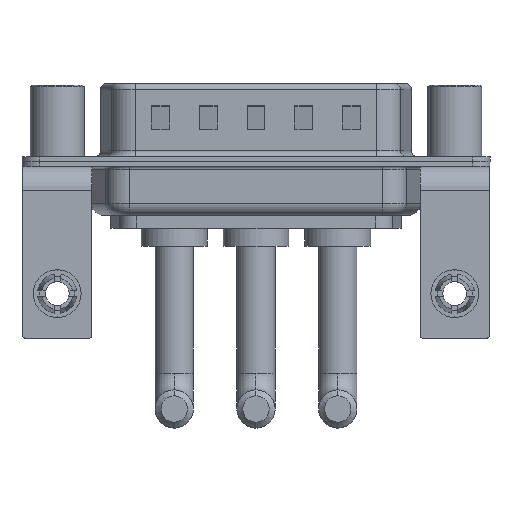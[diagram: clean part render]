
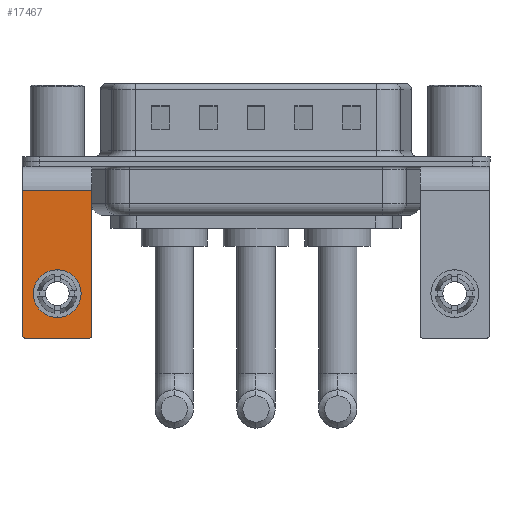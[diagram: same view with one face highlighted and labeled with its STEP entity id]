
A CAD part, front view. The second image highlights one B-rep face of the part: STEP entity #17467.
In plain terms, the highlighted planar face has unit normal (0, -1, 0).
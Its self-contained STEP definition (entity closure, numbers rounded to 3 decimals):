
#400 = DIRECTION ( 'NONE',  ( 0., 0., 1. ) ) ;
#445 = DIRECTION ( 'NONE',  ( -1., 0., 0. ) ) ;
#562 = CARTESIAN_POINT ( 'NONE',  ( -2.9, -6.25, -2.4 ) ) ;
#590 = VECTOR ( 'NONE', #445, 1000. ) ;
#670 = VERTEX_POINT ( 'NONE', #3667 ) ;
#767 = DIRECTION ( 'NONE',  ( 0., 0., 1. ) ) ;
#1478 = CARTESIAN_POINT ( 'NONE',  ( 2.9, -6.25, -2.4 ) ) ;
#1760 = DIRECTION ( 'NONE',  ( 0., 0., 1. ) ) ;
#1906 = PLANE ( 'NONE',  #2375 ) ;
#2089 = ORIENTED_EDGE ( 'NONE', *, *, #6837, .T. ) ;
#2359 = ORIENTED_EDGE ( 'NONE', *, *, #9606, .T. ) ;
#2375 = AXIS2_PLACEMENT_3D ( 'NONE', #9222, #8017, #400 ) ;
#3125 = CIRCLE ( 'NONE', #12724, 2. ) ;
#3216 = FACE_OUTER_BOUND ( 'NONE', #10078, .T. ) ;
#3667 = CARTESIAN_POINT ( 'NONE',  ( 2.65, -6.25, -14.8 ) ) ;
#3905 = DIRECTION ( 'NONE',  ( 0., -1., 0. ) ) ;
#4310 = AXIS2_PLACEMENT_3D ( 'NONE', #9579, #7670, #1760 ) ;
#4416 = CARTESIAN_POINT ( 'NONE',  ( 2.9, -6.25, -14.55 ) ) ;
#4655 = VERTEX_POINT ( 'NONE', #7806 ) ;
#4849 = VECTOR ( 'NONE', #17088, 1000. ) ;
#5169 = ORIENTED_EDGE ( 'NONE', *, *, #8592, .F. ) ;
#5349 = LINE ( 'NONE', #11280, #590 ) ;
#6350 = LINE ( 'NONE', #10973, #4849 ) ;
#6837 = EDGE_CURVE ( 'NONE', #7482, #4655, #9371, .T. ) ;
#7144 = EDGE_CURVE ( 'NONE', #11497, #12368, #6350, .T. ) ;
#7482 = VERTEX_POINT ( 'NONE', #10949 ) ;
#7670 = DIRECTION ( 'NONE',  ( 0., -1., 0. ) ) ;
#7806 = CARTESIAN_POINT ( 'NONE',  ( 0., -6.25, -13.07 ) ) ;
#8017 = DIRECTION ( 'NONE',  ( 0., 1., 0. ) ) ;
#8352 = VERTEX_POINT ( 'NONE', #11073 ) ;
#8592 = EDGE_CURVE ( 'NONE', #670, #19618, #8855, .T. ) ;
#8855 = LINE ( 'NONE', #17887, #18460 ) ;
#8928 = ORIENTED_EDGE ( 'NONE', *, *, #10827, .T. ) ;
#9006 = AXIS2_PLACEMENT_3D ( 'NONE', #12895, #19016, #767 ) ;
#9222 = CARTESIAN_POINT ( 'NONE',  ( 2.9, -6.25, -2.4 ) ) ;
#9371 = CIRCLE ( 'NONE', #9006, 2. ) ;
#9521 = FACE_BOUND ( 'NONE', #15125, .T. ) ;
#9579 = CARTESIAN_POINT ( 'NONE',  ( 2.65, -6.25, -14.55 ) ) ;
#9606 = EDGE_CURVE ( 'NONE', #4655, #7482, #3125, .T. ) ;
#9672 = ORIENTED_EDGE ( 'NONE', *, *, #11397, .T. ) ;
#9826 = DIRECTION ( 'NONE',  ( 0., 0., 1. ) ) ;
#10078 = EDGE_LOOP ( 'NONE', ( #16033, #9672, #5169, #16130, #11704, #8928 ) ) ;
#10827 = EDGE_CURVE ( 'NONE', #11497, #13668, #5349, .T. ) ;
#10949 = CARTESIAN_POINT ( 'NONE',  ( 0., -6.25, -9.07 ) ) ;
#10973 = CARTESIAN_POINT ( 'NONE',  ( 2.9, -6.25, -2.4 ) ) ;
#11073 = CARTESIAN_POINT ( 'NONE',  ( -2.9, -6.25, -14.55 ) ) ;
#11280 = CARTESIAN_POINT ( 'NONE',  ( 2.9, -6.25, -2.4 ) ) ;
#11397 = EDGE_CURVE ( 'NONE', #8352, #19618, #13717, .T. ) ;
#11497 = VERTEX_POINT ( 'NONE', #1478 ) ;
#11704 = ORIENTED_EDGE ( 'NONE', *, *, #7144, .F. ) ;
#12227 = DIRECTION ( 'NONE',  ( 0., 1., 0. ) ) ;
#12368 = VERTEX_POINT ( 'NONE', #4416 ) ;
#12692 = DIRECTION ( 'NONE',  ( 0., 0., -1. ) ) ;
#12724 = AXIS2_PLACEMENT_3D ( 'NONE', #18256, #12227, #16559 ) ;
#12895 = CARTESIAN_POINT ( 'NONE',  ( 0., -6.25, -11.07 ) ) ;
#13668 = VERTEX_POINT ( 'NONE', #16600 ) ;
#13717 = CIRCLE ( 'NONE', #14054, 0.25 ) ;
#14054 = AXIS2_PLACEMENT_3D ( 'NONE', #17649, #3905, #9826 ) ;
#14156 = VECTOR ( 'NONE', #12692, 1000. ) ;
#15125 = EDGE_LOOP ( 'NONE', ( #2359, #2089 ) ) ;
#15470 = EDGE_CURVE ( 'NONE', #13668, #8352, #17517, .T. ) ;
#16033 = ORIENTED_EDGE ( 'NONE', *, *, #15470, .T. ) ;
#16130 = ORIENTED_EDGE ( 'NONE', *, *, #18606, .T. ) ;
#16559 = DIRECTION ( 'NONE',  ( 0., 0., 1. ) ) ;
#16600 = CARTESIAN_POINT ( 'NONE',  ( -2.9, -6.25, -2.4 ) ) ;
#16810 = CIRCLE ( 'NONE', #4310, 0.25 ) ;
#17088 = DIRECTION ( 'NONE',  ( 0., 0., -1. ) ) ;
#17467 = ADVANCED_FACE ( 'NONE', ( #9521, #3216 ), #1906, .F. ) ;
#17517 = LINE ( 'NONE', #562, #14156 ) ;
#17610 = CARTESIAN_POINT ( 'NONE',  ( -2.65, -6.25, -14.8 ) ) ;
#17649 = CARTESIAN_POINT ( 'NONE',  ( -2.65, -6.25, -14.55 ) ) ;
#17887 = CARTESIAN_POINT ( 'NONE',  ( 2.9, -6.25, -14.8 ) ) ;
#18256 = CARTESIAN_POINT ( 'NONE',  ( 0., -6.25, -11.07 ) ) ;
#18460 = VECTOR ( 'NONE', #19571, 1000. ) ;
#18606 = EDGE_CURVE ( 'NONE', #670, #12368, #16810, .T. ) ;
#19016 = DIRECTION ( 'NONE',  ( 0., 1., 0. ) ) ;
#19571 = DIRECTION ( 'NONE',  ( -1., 0., 0. ) ) ;
#19618 = VERTEX_POINT ( 'NONE', #17610 ) ;
